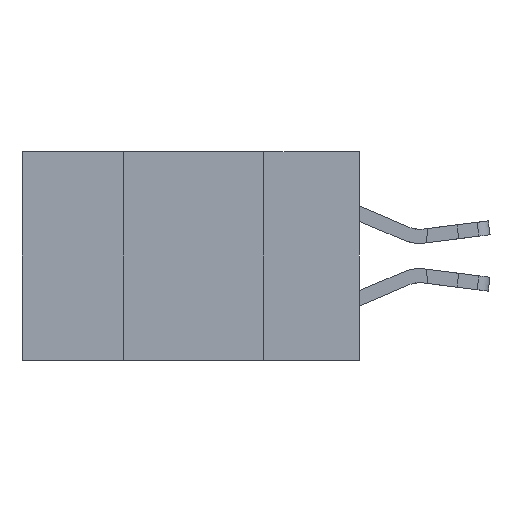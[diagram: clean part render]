
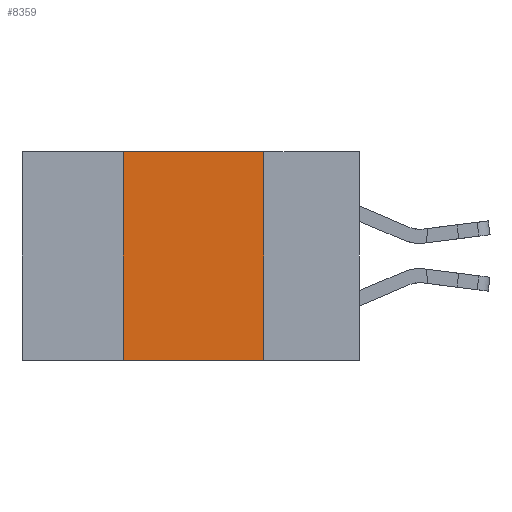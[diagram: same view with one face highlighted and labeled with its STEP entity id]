
A CAD part, left-side view. The second image highlights one B-rep face of the part: STEP entity #8359.
In plain terms, the highlighted planar face has unit normal (-1, 0, 0).
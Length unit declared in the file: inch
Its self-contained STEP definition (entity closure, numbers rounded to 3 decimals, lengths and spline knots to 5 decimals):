
#287 = VECTOR ( 'NONE', #2255, 39.37008 ) ;
#523 = DIRECTION ( 'NONE',  ( 0., 0., -1. ) ) ;
#1583 = EDGE_CURVE ( 'NONE', #1638, #17840, #14679, .T. ) ;
#1638 = VERTEX_POINT ( 'NONE', #10394 ) ;
#1690 = CARTESIAN_POINT ( 'NONE',  ( 0., 0.6, 0. ) ) ;
#2255 = DIRECTION ( 'NONE',  ( 0., 0., 1. ) ) ;
#2973 = DIRECTION ( 'NONE',  ( 0., -1., 0. ) ) ;
#2976 = EDGE_CURVE ( 'NONE', #20280, #10380, #5431, .T. ) ;
#2981 = AXIS2_PLACEMENT_3D ( 'NONE', #1690, #23296, #12304 ) ;
#3130 = CARTESIAN_POINT ( 'NONE',  ( 0., 0.6, -0.37 ) ) ;
#4189 = VECTOR ( 'NONE', #523, 39.37008 ) ;
#5326 = LINE ( 'NONE', #8023, #4189 ) ;
#5431 = LINE ( 'NONE', #20683, #11436 ) ;
#5782 = VECTOR ( 'NONE', #2973, 39.37008 ) ;
#5866 = EDGE_CURVE ( 'NONE', #1638, #20280, #13453, .T. ) ;
#8023 = CARTESIAN_POINT ( 'NONE',  ( 0., 0.17, 0. ) ) ;
#8359 = ADVANCED_FACE ( 'NONE', ( #22570 ), #21792, .F. ) ;
#8609 = CARTESIAN_POINT ( 'NONE',  ( 0., 0.17, 0. ) ) ;
#8797 = CARTESIAN_POINT ( 'NONE',  ( 0., 0.42, 0. ) ) ;
#10380 = VERTEX_POINT ( 'NONE', #8609 ) ;
#10394 = CARTESIAN_POINT ( 'NONE',  ( 0., 0.42, -0.37 ) ) ;
#10440 = ORIENTED_EDGE ( 'NONE', *, *, #12419, .F. ) ;
#10646 = ORIENTED_EDGE ( 'NONE', *, *, #1583, .T. ) ;
#11436 = VECTOR ( 'NONE', #11481, 39.37008 ) ;
#11481 = DIRECTION ( 'NONE',  ( 0., -1., 0. ) ) ;
#12304 = DIRECTION ( 'NONE',  ( 0., 0., -1. ) ) ;
#12419 = EDGE_CURVE ( 'NONE', #10380, #17840, #5326, .T. ) ;
#13115 = CARTESIAN_POINT ( 'NONE',  ( 0., 0.42, 0. ) ) ;
#13230 = CARTESIAN_POINT ( 'NONE',  ( 0., 0.17, -0.37 ) ) ;
#13453 = LINE ( 'NONE', #13115, #287 ) ;
#13497 = ORIENTED_EDGE ( 'NONE', *, *, #2976, .F. ) ;
#14679 = LINE ( 'NONE', #3130, #5782 ) ;
#17840 = VERTEX_POINT ( 'NONE', #13230 ) ;
#19416 = ORIENTED_EDGE ( 'NONE', *, *, #5866, .F. ) ;
#20280 = VERTEX_POINT ( 'NONE', #8797 ) ;
#20683 = CARTESIAN_POINT ( 'NONE',  ( 0., 0.6, 0. ) ) ;
#21792 = PLANE ( 'NONE',  #2981 ) ;
#22570 = FACE_OUTER_BOUND ( 'NONE', #23328, .T. ) ;
#23296 = DIRECTION ( 'NONE',  ( 1., 0., 0. ) ) ;
#23328 = EDGE_LOOP ( 'NONE', ( #10440, #13497, #19416, #10646 ) ) ;
